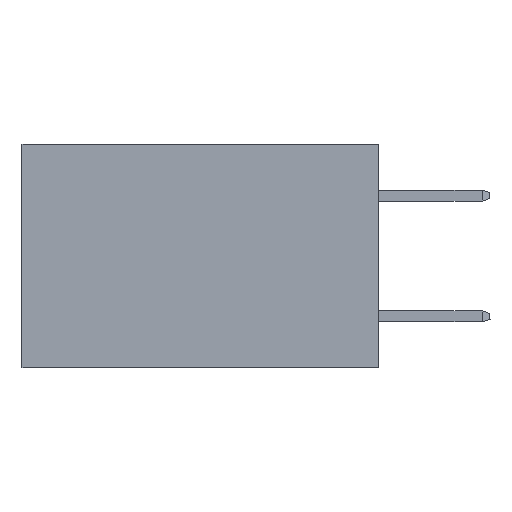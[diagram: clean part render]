
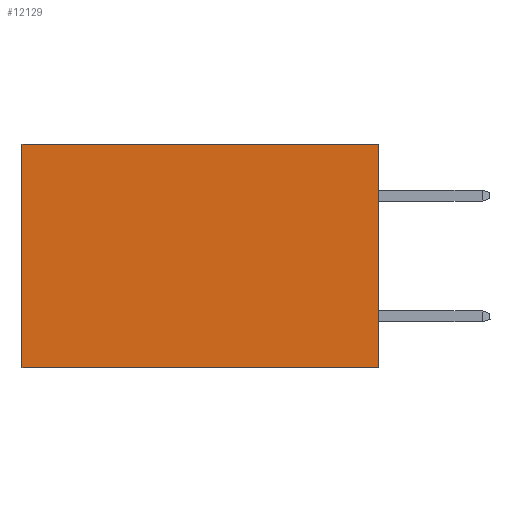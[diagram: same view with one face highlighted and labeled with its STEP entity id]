
A CAD part, left-side view. The second image highlights one B-rep face of the part: STEP entity #12129.
In plain terms, the highlighted planar face has unit normal (-1, 0, 0).
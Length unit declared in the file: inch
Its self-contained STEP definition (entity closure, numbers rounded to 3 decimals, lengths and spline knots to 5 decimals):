
#641 = DIRECTION ( 'NONE',  ( 0., 1., 0. ) ) ;
#902 = CARTESIAN_POINT ( 'NONE',  ( 0.277, 0., -0.37 ) ) ;
#1531 = EDGE_CURVE ( 'NONE', #12095, #3046, #21774, .T. ) ;
#1734 = VERTEX_POINT ( 'NONE', #4301 ) ;
#1906 = VECTOR ( 'NONE', #9114, 39.37008 ) ;
#2505 = CARTESIAN_POINT ( 'NONE',  ( 0.277, 0.59, -0.37 ) ) ;
#2593 = LINE ( 'NONE', #19850, #1906 ) ;
#3046 = VERTEX_POINT ( 'NONE', #6453 ) ;
#4301 = CARTESIAN_POINT ( 'NONE',  ( 0.277, 0.59, 0. ) ) ;
#4509 = EDGE_LOOP ( 'NONE', ( #9582, #10083, #12041, #12393 ) ) ;
#4924 = DIRECTION ( 'NONE',  ( 0., 0., -1. ) ) ;
#5091 = EDGE_CURVE ( 'NONE', #12095, #1734, #24064, .T. ) ;
#5269 = CARTESIAN_POINT ( 'NONE',  ( 0.277, 0., -0.37 ) ) ;
#6453 = CARTESIAN_POINT ( 'NONE',  ( 0.277, 0., -0.37 ) ) ;
#7005 = VECTOR ( 'NONE', #9002, 39.37008 ) ;
#7246 = FACE_OUTER_BOUND ( 'NONE', #4509, .T. ) ;
#9002 = DIRECTION ( 'NONE',  ( 0., 1., 0. ) ) ;
#9114 = DIRECTION ( 'NONE',  ( 0., 0., -1. ) ) ;
#9496 = PLANE ( 'NONE',  #26345 ) ;
#9582 = ORIENTED_EDGE ( 'NONE', *, *, #10491, .T. ) ;
#9587 = DIRECTION ( 'NONE',  ( 0., 0., -1. ) ) ;
#10083 = ORIENTED_EDGE ( 'NONE', *, *, #10247, .F. ) ;
#10247 = EDGE_CURVE ( 'NONE', #3046, #16756, #25337, .T. ) ;
#10491 = EDGE_CURVE ( 'NONE', #1734, #16756, #2593, .T. ) ;
#11392 = CARTESIAN_POINT ( 'NONE',  ( 0.277, 0., 0. ) ) ;
#12041 = ORIENTED_EDGE ( 'NONE', *, *, #1531, .F. ) ;
#12095 = VERTEX_POINT ( 'NONE', #26487 ) ;
#12129 = ADVANCED_FACE ( 'NONE', ( #7246 ), #9496, .F. ) ;
#12393 = ORIENTED_EDGE ( 'NONE', *, *, #5091, .T. ) ;
#13987 = VECTOR ( 'NONE', #641, 39.37008 ) ;
#16019 = VECTOR ( 'NONE', #4924, 39.37008 ) ;
#16756 = VERTEX_POINT ( 'NONE', #2505 ) ;
#17572 = CARTESIAN_POINT ( 'NONE',  ( 0.277, 0., -0.37 ) ) ;
#19850 = CARTESIAN_POINT ( 'NONE',  ( 0.277, 0.59, -0.37 ) ) ;
#21774 = LINE ( 'NONE', #17572, #16019 ) ;
#22454 = DIRECTION ( 'NONE',  ( 1., 0., 0. ) ) ;
#24064 = LINE ( 'NONE', #11392, #7005 ) ;
#25337 = LINE ( 'NONE', #902, #13987 ) ;
#26345 = AXIS2_PLACEMENT_3D ( 'NONE', #5269, #22454, #9587 ) ;
#26487 = CARTESIAN_POINT ( 'NONE',  ( 0.277, 0., 0. ) ) ;
